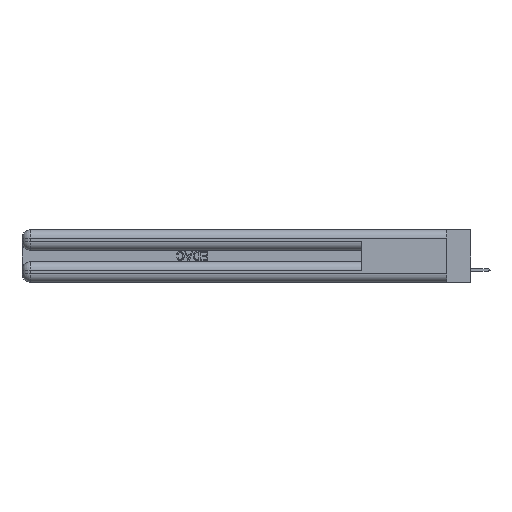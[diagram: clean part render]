
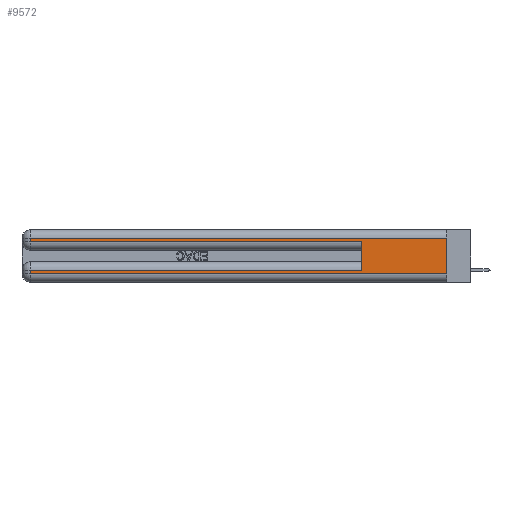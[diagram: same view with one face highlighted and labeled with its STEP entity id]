
A CAD part, left-side view. The second image highlights one B-rep face of the part: STEP entity #9572.
In plain terms, the highlighted planar face has unit normal (-1, 0, 0).
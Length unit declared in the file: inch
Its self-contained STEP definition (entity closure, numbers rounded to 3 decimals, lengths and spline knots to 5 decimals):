
#80 = CARTESIAN_POINT ( 'NONE',  ( 0., 2.94, 0.37 ) ) ;
#937 = VECTOR ( 'NONE', #27645, 39.37008 ) ;
#1058 = LINE ( 'NONE', #20662, #42241 ) ;
#1158 = VECTOR ( 'NONE', #26347, 39.37008 ) ;
#1778 = VERTEX_POINT ( 'NONE', #17695 ) ;
#3385 = ORIENTED_EDGE ( 'NONE', *, *, #19466, .T. ) ;
#3783 = CARTESIAN_POINT ( 'NONE',  ( 0., 0.6, 0.285 ) ) ;
#4292 = DIRECTION ( 'NONE',  ( 0., 1., 0. ) ) ;
#4742 = CARTESIAN_POINT ( 'NONE',  ( 0., 2.94, 0.085 ) ) ;
#4908 = EDGE_CURVE ( 'NONE', #17339, #7387, #23159, .T. ) ;
#4993 = DIRECTION ( 'NONE',  ( 1., 0., 0. ) ) ;
#5366 = VERTEX_POINT ( 'NONE', #9782 ) ;
#5941 = CARTESIAN_POINT ( 'NONE',  ( 0., 0.6, 0.145 ) ) ;
#6985 = VECTOR ( 'NONE', #25922, 39.37008 ) ;
#7387 = VERTEX_POINT ( 'NONE', #21536 ) ;
#8550 = EDGE_CURVE ( 'NONE', #5366, #39111, #23477, .T. ) ;
#9137 = ORIENTED_EDGE ( 'NONE', *, *, #4908, .T. ) ;
#9572 = ADVANCED_FACE ( 'NONE', ( #37084 ), #11239, .F. ) ;
#9782 = CARTESIAN_POINT ( 'NONE',  ( 0., 2.94, 0.285 ) ) ;
#10635 = EDGE_CURVE ( 'NONE', #1778, #39111, #23381, .T. ) ;
#10948 = ORIENTED_EDGE ( 'NONE', *, *, #34186, .F. ) ;
#11125 = VERTEX_POINT ( 'NONE', #4742 ) ;
#11239 = PLANE ( 'NONE',  #30947 ) ;
#12439 = CARTESIAN_POINT ( 'NONE',  ( 0., 2.94, 0.06 ) ) ;
#12782 = CARTESIAN_POINT ( 'NONE',  ( 0., 0., 0.37 ) ) ;
#15351 = ORIENTED_EDGE ( 'NONE', *, *, #30695, .T. ) ;
#15928 = EDGE_CURVE ( 'NONE', #27881, #5366, #19288, .T. ) ;
#16058 = DIRECTION ( 'NONE',  ( 0., -1., 0. ) ) ;
#16455 = VECTOR ( 'NONE', #42224, 39.37008 ) ;
#16775 = VECTOR ( 'NONE', #19069, 39.37008 ) ;
#17339 = VERTEX_POINT ( 'NONE', #12439 ) ;
#17695 = CARTESIAN_POINT ( 'NONE',  ( 0., 0.6, 0.085 ) ) ;
#18119 = DIRECTION ( 'NONE',  ( 0., 0., -1. ) ) ;
#19069 = DIRECTION ( 'NONE',  ( 0., 0., -1. ) ) ;
#19070 = DIRECTION ( 'NONE',  ( 0., 0., 1. ) ) ;
#19288 = LINE ( 'NONE', #35450, #16775 ) ;
#19466 = EDGE_CURVE ( 'NONE', #11125, #17339, #29583, .T. ) ;
#20034 = CARTESIAN_POINT ( 'NONE',  ( 0., 0., 0.285 ) ) ;
#20662 = CARTESIAN_POINT ( 'NONE',  ( 0., 0., 0.31 ) ) ;
#21185 = CARTESIAN_POINT ( 'NONE',  ( 0., 0., 0.085 ) ) ;
#21362 = CARTESIAN_POINT ( 'NONE',  ( 0., 0., 0.37 ) ) ;
#21536 = CARTESIAN_POINT ( 'NONE',  ( 0., 0., 0.06 ) ) ;
#23159 = LINE ( 'NONE', #29414, #30124 ) ;
#23381 = LINE ( 'NONE', #5941, #31596 ) ;
#23477 = LINE ( 'NONE', #20034, #16455 ) ;
#25922 = DIRECTION ( 'NONE',  ( 0., 0., -1. ) ) ;
#26347 = DIRECTION ( 'NONE',  ( 0., 0., -1. ) ) ;
#27645 = DIRECTION ( 'NONE',  ( 0., 1., 0. ) ) ;
#27647 = ORIENTED_EDGE ( 'NONE', *, *, #10635, .F. ) ;
#27881 = VERTEX_POINT ( 'NONE', #38813 ) ;
#28013 = ORIENTED_EDGE ( 'NONE', *, *, #15928, .T. ) ;
#29414 = CARTESIAN_POINT ( 'NONE',  ( 0., 0., 0.06 ) ) ;
#29583 = LINE ( 'NONE', #80, #1158 ) ;
#30124 = VECTOR ( 'NONE', #16058, 39.37008 ) ;
#30695 = EDGE_CURVE ( 'NONE', #1778, #11125, #30874, .T. ) ;
#30874 = LINE ( 'NONE', #21185, #937 ) ;
#30947 = AXIS2_PLACEMENT_3D ( 'NONE', #21362, #4993, #18119 ) ;
#31284 = ORIENTED_EDGE ( 'NONE', *, *, #8550, .T. ) ;
#31596 = VECTOR ( 'NONE', #19070, 39.37008 ) ;
#32673 = ORIENTED_EDGE ( 'NONE', *, *, #37038, .T. ) ;
#34186 = EDGE_CURVE ( 'NONE', #38197, #7387, #42077, .T. ) ;
#35450 = CARTESIAN_POINT ( 'NONE',  ( 0., 2.94, 0.37 ) ) ;
#37038 = EDGE_CURVE ( 'NONE', #38197, #27881, #1058, .T. ) ;
#37084 = FACE_OUTER_BOUND ( 'NONE', #41192, .T. ) ;
#38197 = VERTEX_POINT ( 'NONE', #42291 ) ;
#38813 = CARTESIAN_POINT ( 'NONE',  ( 0., 2.94, 0.31 ) ) ;
#39111 = VERTEX_POINT ( 'NONE', #3783 ) ;
#41192 = EDGE_LOOP ( 'NONE', ( #10948, #32673, #28013, #31284, #27647, #15351, #3385, #9137 ) ) ;
#42077 = LINE ( 'NONE', #12782, #6985 ) ;
#42224 = DIRECTION ( 'NONE',  ( 0., -1., 0. ) ) ;
#42241 = VECTOR ( 'NONE', #4292, 39.37008 ) ;
#42291 = CARTESIAN_POINT ( 'NONE',  ( 0., 0., 0.31 ) ) ;
